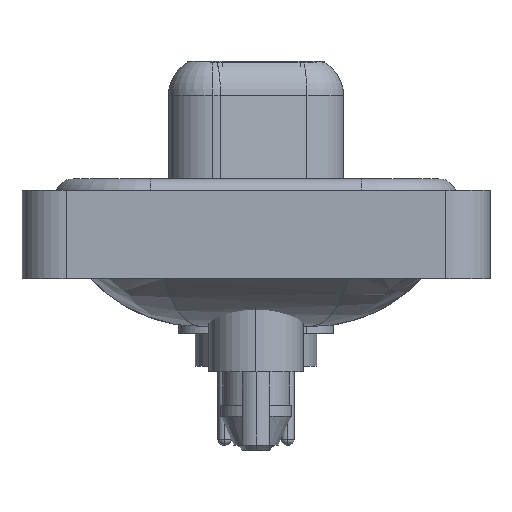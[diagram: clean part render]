
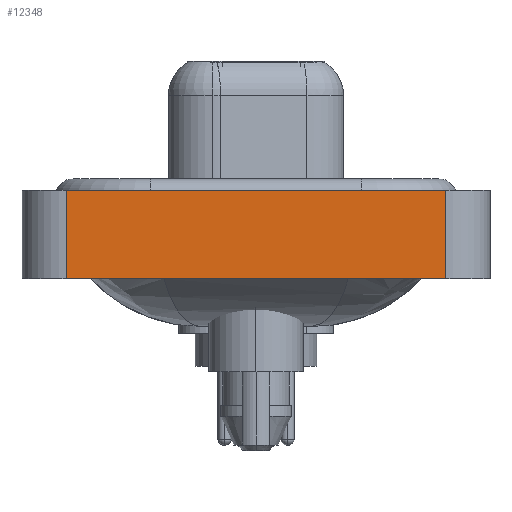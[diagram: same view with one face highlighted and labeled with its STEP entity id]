
A CAD part, left-side view. The second image highlights one B-rep face of the part: STEP entity #12348.
In plain terms, the highlighted planar face has unit normal (-1, 0, 0).
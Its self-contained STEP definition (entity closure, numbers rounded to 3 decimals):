
#974 = CARTESIAN_POINT ( 'NONE',  ( -7.35, 8.55, -3.6 ) ) ;
#1092 = CARTESIAN_POINT ( 'NONE',  ( -7.35, -8.55, 0.4 ) ) ;
#1470 = PLANE ( 'NONE',  #3791 ) ;
#1549 = CARTESIAN_POINT ( 'NONE',  ( -7.35, 8.55, 0.4 ) ) ;
#2723 = VERTEX_POINT ( 'NONE', #20004 ) ;
#3283 = DIRECTION ( 'NONE',  ( -1., 0., 0. ) ) ;
#3791 = AXIS2_PLACEMENT_3D ( 'NONE', #5220, #3283, #18694 ) ;
#4252 = ORIENTED_EDGE ( 'NONE', *, *, #11253, .T. ) ;
#4424 = LINE ( 'NONE', #19842, #4461 ) ;
#4461 = VECTOR ( 'NONE', #16213, 1000. ) ;
#5220 = CARTESIAN_POINT ( 'NONE',  ( -7.35, -8.55, -3.6 ) ) ;
#5243 = VERTEX_POINT ( 'NONE', #1092 ) ;
#5306 = EDGE_CURVE ( 'NONE', #2723, #5243, #18770, .T. ) ;
#6301 = VECTOR ( 'NONE', #20245, 1000. ) ;
#6469 = CARTESIAN_POINT ( 'NONE',  ( -7.35, 8.55, -3.6 ) ) ;
#8010 = LINE ( 'NONE', #974, #6301 ) ;
#8237 = ORIENTED_EDGE ( 'NONE', *, *, #20134, .F. ) ;
#9968 = VERTEX_POINT ( 'NONE', #1549 ) ;
#11253 = EDGE_CURVE ( 'NONE', #19370, #2723, #4424, .T. ) ;
#11639 = ORIENTED_EDGE ( 'NONE', *, *, #5306, .T. ) ;
#12348 = ADVANCED_FACE ( 'NONE', ( #16984 ), #1470, .T. ) ;
#12457 = ORIENTED_EDGE ( 'NONE', *, *, #14959, .F. ) ;
#14959 = EDGE_CURVE ( 'NONE', #19370, #9968, #8010, .T. ) ;
#15376 = CARTESIAN_POINT ( 'NONE',  ( -7.35, -8.55, -3.6 ) ) ;
#16213 = DIRECTION ( 'NONE',  ( 0., -1., 0. ) ) ;
#16984 = FACE_OUTER_BOUND ( 'NONE', #17090, .T. ) ;
#17090 = EDGE_LOOP ( 'NONE', ( #11639, #8237, #12457, #4252 ) ) ;
#17399 = DIRECTION ( 'NONE',  ( 0., -1., 0. ) ) ;
#17448 = VECTOR ( 'NONE', #17399, 1000. ) ;
#17680 = VECTOR ( 'NONE', #18430, 1000. ) ;
#17730 = CARTESIAN_POINT ( 'NONE',  ( -7.35, -8.55, 0.4 ) ) ;
#18430 = DIRECTION ( 'NONE',  ( 0., 0., 1. ) ) ;
#18694 = DIRECTION ( 'NONE',  ( 0., 0., 1. ) ) ;
#18770 = LINE ( 'NONE', #15376, #17680 ) ;
#19370 = VERTEX_POINT ( 'NONE', #6469 ) ;
#19842 = CARTESIAN_POINT ( 'NONE',  ( -7.35, -8.55, -3.6 ) ) ;
#20004 = CARTESIAN_POINT ( 'NONE',  ( -7.35, -8.55, -3.6 ) ) ;
#20134 = EDGE_CURVE ( 'NONE', #9968, #5243, #21027, .T. ) ;
#20245 = DIRECTION ( 'NONE',  ( 0., 0., 1. ) ) ;
#21027 = LINE ( 'NONE', #17730, #17448 ) ;
